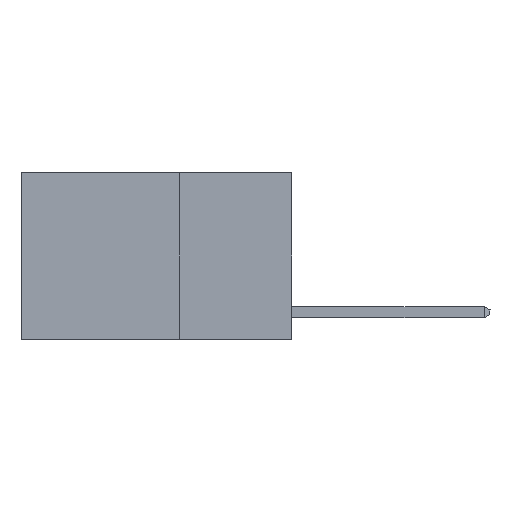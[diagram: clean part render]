
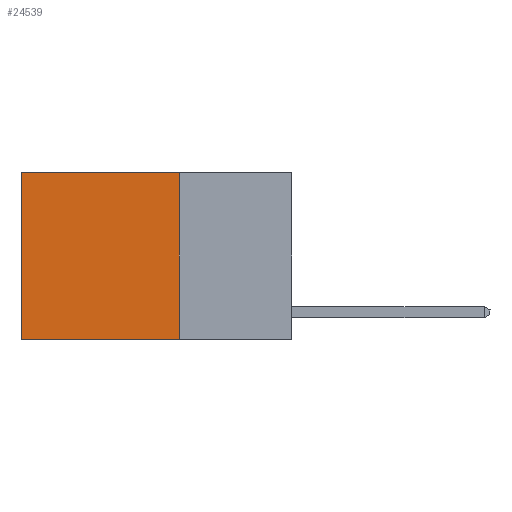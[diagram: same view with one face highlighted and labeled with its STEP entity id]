
A CAD part, left-side view. The second image highlights one B-rep face of the part: STEP entity #24539.
In plain terms, the highlighted planar face has unit normal (-1, 0, 0).
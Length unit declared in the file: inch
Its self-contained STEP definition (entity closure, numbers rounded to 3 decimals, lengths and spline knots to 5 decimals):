
#1492 = CARTESIAN_POINT ( 'NONE',  ( 0.2625, 0.25, -0.37 ) ) ;
#2641 = CARTESIAN_POINT ( 'NONE',  ( 0.2625, 0.25, -0.37 ) ) ;
#2708 = ORIENTED_EDGE ( 'NONE', *, *, #6233, .T. ) ;
#3377 = CARTESIAN_POINT ( 'NONE',  ( 0.2625, 0.25, 0. ) ) ;
#5423 = ORIENTED_EDGE ( 'NONE', *, *, #7218, .F. ) ;
#5507 = VERTEX_POINT ( 'NONE', #2641 ) ;
#6233 = EDGE_CURVE ( 'NONE', #20909, #11385, #22426, .T. ) ;
#7218 = EDGE_CURVE ( 'NONE', #20909, #5507, #23780, .T. ) ;
#8035 = CARTESIAN_POINT ( 'NONE',  ( 0.2625, 0.6, 0. ) ) ;
#8237 = EDGE_LOOP ( 'NONE', ( #25266, #16874, #5423, #2708 ) ) ;
#8848 = DIRECTION ( 'NONE',  ( 1., 0., 0. ) ) ;
#9149 = VECTOR ( 'NONE', #19626, 39.37008 ) ;
#9317 = VECTOR ( 'NONE', #27136, 39.37008 ) ;
#11198 = AXIS2_PLACEMENT_3D ( 'NONE', #20120, #8848, #17954 ) ;
#11245 = VERTEX_POINT ( 'NONE', #18425 ) ;
#11385 = VERTEX_POINT ( 'NONE', #14341 ) ;
#11904 = EDGE_CURVE ( 'NONE', #11385, #11245, #20114, .T. ) ;
#14341 = CARTESIAN_POINT ( 'NONE',  ( 0.2625, 0.6, 0. ) ) ;
#14930 = CARTESIAN_POINT ( 'NONE',  ( 0.2625, 0.25, 0. ) ) ;
#16874 = ORIENTED_EDGE ( 'NONE', *, *, #29159, .F. ) ;
#17850 = PLANE ( 'NONE',  #11198 ) ;
#17954 = DIRECTION ( 'NONE',  ( 0., 0., -1. ) ) ;
#18425 = CARTESIAN_POINT ( 'NONE',  ( 0.2625, 0.6, -0.37 ) ) ;
#18677 = FACE_OUTER_BOUND ( 'NONE', #8237, .T. ) ;
#19353 = DIRECTION ( 'NONE',  ( 0., 0., -1. ) ) ;
#19626 = DIRECTION ( 'NONE',  ( 0., 1., 0. ) ) ;
#20114 = LINE ( 'NONE', #8035, #20454 ) ;
#20120 = CARTESIAN_POINT ( 'NONE',  ( 0.2625, 0.25, 0. ) ) ;
#20454 = VECTOR ( 'NONE', #28859, 39.37008 ) ;
#20909 = VERTEX_POINT ( 'NONE', #14930 ) ;
#22426 = LINE ( 'NONE', #22690, #9317 ) ;
#22690 = CARTESIAN_POINT ( 'NONE',  ( 0.2625, 0.25, 0. ) ) ;
#23780 = LINE ( 'NONE', #3377, #29120 ) ;
#24539 = ADVANCED_FACE ( 'NONE', ( #18677 ), #17850, .F. ) ;
#25266 = ORIENTED_EDGE ( 'NONE', *, *, #11904, .T. ) ;
#27136 = DIRECTION ( 'NONE',  ( 0., 1., 0. ) ) ;
#27927 = LINE ( 'NONE', #1492, #9149 ) ;
#28859 = DIRECTION ( 'NONE',  ( 0., 0., -1. ) ) ;
#29120 = VECTOR ( 'NONE', #19353, 39.37008 ) ;
#29159 = EDGE_CURVE ( 'NONE', #5507, #11245, #27927, .T. ) ;
